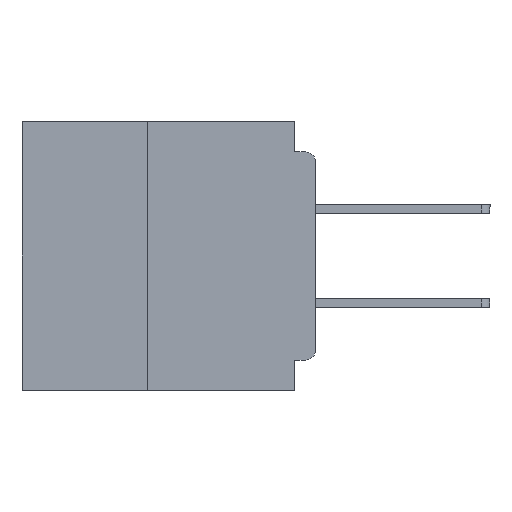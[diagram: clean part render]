
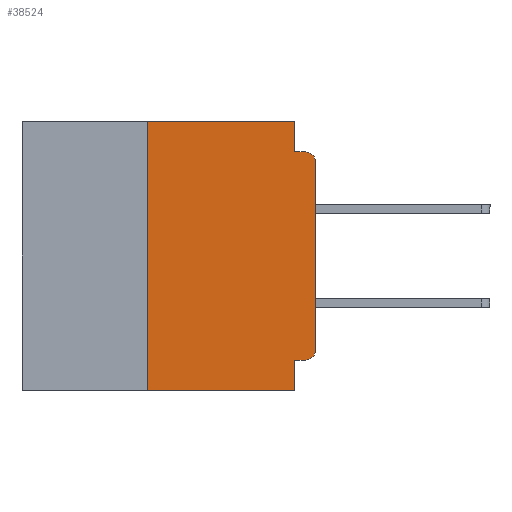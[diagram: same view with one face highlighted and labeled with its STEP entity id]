
A CAD part, left-side view. The second image highlights one B-rep face of the part: STEP entity #38524.
In plain terms, the highlighted planar face has unit normal (-1, 0, 0).
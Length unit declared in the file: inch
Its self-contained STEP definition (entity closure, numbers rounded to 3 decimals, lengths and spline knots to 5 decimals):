
#200 = DIRECTION ( 'NONE',  ( 0., 0., -1. ) ) ;
#320 = CIRCLE ( 'NONE', #39752, 0.015 ) ;
#388 = VERTEX_POINT ( 'NONE', #32232 ) ;
#759 = DIRECTION ( 'NONE',  ( -1., 0., 0. ) ) ;
#835 = FACE_OUTER_BOUND ( 'NONE', #11242, .T. ) ;
#1042 = ORIENTED_EDGE ( 'NONE', *, *, #27322, .T. ) ;
#1289 = DIRECTION ( 'NONE',  ( -1., 0., 0. ) ) ;
#1573 = VERTEX_POINT ( 'NONE', #11454 ) ;
#1989 = EDGE_CURVE ( 'NONE', #21328, #25784, #18048, .T. ) ;
#3049 = VECTOR ( 'NONE', #200, 39.37008 ) ;
#3705 = LINE ( 'NONE', #27062, #37245 ) ;
#4581 = CARTESIAN_POINT ( 'NONE',  ( 0., 0.031, -0.355 ) ) ;
#5218 = EDGE_CURVE ( 'NONE', #40222, #1573, #17297, .T. ) ;
#6237 = ORIENTED_EDGE ( 'NONE', *, *, #15723, .T. ) ;
#6256 = DIRECTION ( 'NONE',  ( 0., 0., 1. ) ) ;
#6490 = CIRCLE ( 'NONE', #18163, 0.015 ) ;
#6608 = EDGE_CURVE ( 'NONE', #31339, #18027, #38454, .T. ) ;
#10189 = LINE ( 'NONE', #10692, #26375 ) ;
#10692 = CARTESIAN_POINT ( 'NONE',  ( 0., 0., -0.355 ) ) ;
#10806 = LINE ( 'NONE', #23142, #3049 ) ;
#11242 = EDGE_LOOP ( 'NONE', ( #13965, #6237, #33182, #17029, #36190, #20052, #23097, #40281, #25075, #1042 ) ) ;
#11454 = CARTESIAN_POINT ( 'NONE',  ( 0., 0.031, -0.4 ) ) ;
#11959 = LINE ( 'NONE', #38241, #29152 ) ;
#13416 = VERTEX_POINT ( 'NONE', #36468 ) ;
#13965 = ORIENTED_EDGE ( 'NONE', *, *, #1989, .T. ) ;
#14007 = DIRECTION ( 'NONE',  ( 0., 1., 0. ) ) ;
#14249 = DIRECTION ( 'NONE',  ( 0., -1., 0. ) ) ;
#14608 = EDGE_CURVE ( 'NONE', #30260, #13416, #10806, .T. ) ;
#15656 = DIRECTION ( 'NONE',  ( 0., -1., 0. ) ) ;
#15723 = EDGE_CURVE ( 'NONE', #25784, #35412, #320, .T. ) ;
#17029 = ORIENTED_EDGE ( 'NONE', *, *, #14608, .F. ) ;
#17297 = LINE ( 'NONE', #34219, #42056 ) ;
#18027 = VERTEX_POINT ( 'NONE', #28993 ) ;
#18048 = LINE ( 'NONE', #40983, #36246 ) ;
#18163 = AXIS2_PLACEMENT_3D ( 'NONE', #20941, #1289, #24194 ) ;
#18986 = EDGE_CURVE ( 'NONE', #18027, #30260, #38097, .T. ) ;
#19167 = DIRECTION ( 'NONE',  ( 1., 0., 0. ) ) ;
#20052 = ORIENTED_EDGE ( 'NONE', *, *, #6608, .F. ) ;
#20427 = CARTESIAN_POINT ( 'NONE',  ( 0., 0.015, -0.06 ) ) ;
#20941 = CARTESIAN_POINT ( 'NONE',  ( 0., 0.015, -0.34 ) ) ;
#21258 = VECTOR ( 'NONE', #6256, 39.37008 ) ;
#21328 = VERTEX_POINT ( 'NONE', #36150 ) ;
#23097 = ORIENTED_EDGE ( 'NONE', *, *, #42210, .T. ) ;
#23142 = CARTESIAN_POINT ( 'NONE',  ( 0., 0.031, 0. ) ) ;
#23696 = DIRECTION ( 'NONE',  ( 0., 0., -1. ) ) ;
#23790 = DIRECTION ( 'NONE',  ( 0., -1., 0. ) ) ;
#24127 = EDGE_CURVE ( 'NONE', #13416, #35412, #11959, .T. ) ;
#24194 = DIRECTION ( 'NONE',  ( 0., 0., -1. ) ) ;
#24434 = CARTESIAN_POINT ( 'NONE',  ( 0., 0.031, 0. ) ) ;
#25075 = ORIENTED_EDGE ( 'NONE', *, *, #30092, .F. ) ;
#25784 = VERTEX_POINT ( 'NONE', #34405 ) ;
#26375 = VECTOR ( 'NONE', #14007, 39.37008 ) ;
#26842 = CARTESIAN_POINT ( 'NONE',  ( 0., 0.25, -0.4 ) ) ;
#27062 = CARTESIAN_POINT ( 'NONE',  ( 0., 0.437, -0.4 ) ) ;
#27322 = EDGE_CURVE ( 'NONE', #388, #21328, #6490, .T. ) ;
#28478 = VECTOR ( 'NONE', #23790, 39.37008 ) ;
#28993 = CARTESIAN_POINT ( 'NONE',  ( 0., 0.25, 0. ) ) ;
#29152 = VECTOR ( 'NONE', #15656, 39.37008 ) ;
#30092 = EDGE_CURVE ( 'NONE', #388, #40222, #10189, .T. ) ;
#30260 = VERTEX_POINT ( 'NONE', #24434 ) ;
#30277 = CARTESIAN_POINT ( 'NONE',  ( 0., 0.437, 0. ) ) ;
#31339 = VERTEX_POINT ( 'NONE', #26842 ) ;
#32057 = CARTESIAN_POINT ( 'NONE',  ( 0., 0.437, 0. ) ) ;
#32232 = CARTESIAN_POINT ( 'NONE',  ( 0., 0.015, -0.355 ) ) ;
#33182 = ORIENTED_EDGE ( 'NONE', *, *, #24127, .F. ) ;
#34037 = DIRECTION ( 'NONE',  ( 0., 0., -1. ) ) ;
#34219 = CARTESIAN_POINT ( 'NONE',  ( 0., 0.031, -0.4 ) ) ;
#34405 = CARTESIAN_POINT ( 'NONE',  ( 0., 0., -0.06 ) ) ;
#35412 = VERTEX_POINT ( 'NONE', #36530 ) ;
#35487 = CARTESIAN_POINT ( 'NONE',  ( 0., 0.25, -0.4 ) ) ;
#36150 = CARTESIAN_POINT ( 'NONE',  ( 0., 0., -0.34 ) ) ;
#36190 = ORIENTED_EDGE ( 'NONE', *, *, #18986, .F. ) ;
#36246 = VECTOR ( 'NONE', #41376, 39.37008 ) ;
#36468 = CARTESIAN_POINT ( 'NONE',  ( 0., 0.031, -0.045 ) ) ;
#36530 = CARTESIAN_POINT ( 'NONE',  ( 0., 0.015, -0.045 ) ) ;
#37245 = VECTOR ( 'NONE', #14249, 39.37008 ) ;
#38097 = LINE ( 'NONE', #30277, #28478 ) ;
#38241 = CARTESIAN_POINT ( 'NONE',  ( 0., 0., -0.045 ) ) ;
#38454 = LINE ( 'NONE', #35487, #21258 ) ;
#38524 = ADVANCED_FACE ( 'NONE', ( #835 ), #38525, .F. ) ;
#38525 = PLANE ( 'NONE',  #39366 ) ;
#39366 = AXIS2_PLACEMENT_3D ( 'NONE', #32057, #19167, #41792 ) ;
#39752 = AXIS2_PLACEMENT_3D ( 'NONE', #20427, #759, #23696 ) ;
#40222 = VERTEX_POINT ( 'NONE', #4581 ) ;
#40281 = ORIENTED_EDGE ( 'NONE', *, *, #5218, .F. ) ;
#40983 = CARTESIAN_POINT ( 'NONE',  ( 0., 0., 0. ) ) ;
#41376 = DIRECTION ( 'NONE',  ( 0., 0., 1. ) ) ;
#41792 = DIRECTION ( 'NONE',  ( 0., 0., -1. ) ) ;
#42056 = VECTOR ( 'NONE', #34037, 39.37008 ) ;
#42210 = EDGE_CURVE ( 'NONE', #31339, #1573, #3705, .T. ) ;
